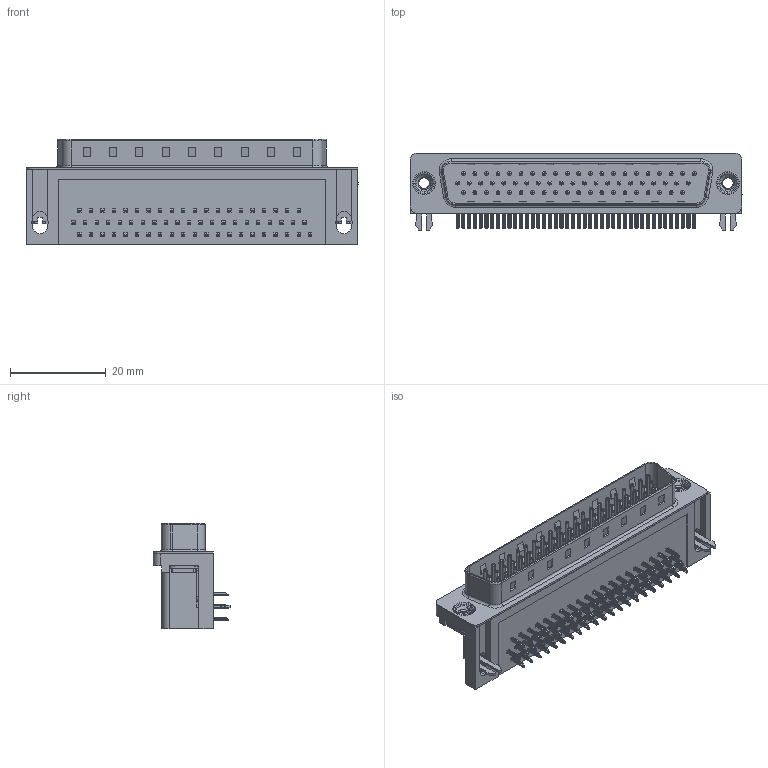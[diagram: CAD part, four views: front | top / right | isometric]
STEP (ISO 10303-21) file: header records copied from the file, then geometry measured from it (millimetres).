
FILE_DESCRIPTION (( 'STEP AP203' ), '1' );
FILE_NAME ('633-062-263-032.STEP', '2018-09-07T21:38:47', ( '' ), ( '' ), 'SwSTEP 2.0', 'SolidWorks 2016', '' );
FILE_SCHEMA (( 'CONFIG_CONTROL_DESIGN' ));
Length unit declared in the file: millimetre
Products named in the file (8): 633 2 Prong Board Lock; 633 4-40 Threaded Rivet; 633-062-263-032; 633 Housing_62 Contact; 633 Shell_62 Contact; 633 Contact Bottom; 633 Contact Middle; 633 Contact Top
Assembly tree (68 placements, depth 2):
  633-062-263-032
    633 Housing_62 Contact
    633 Shell_62 Contact
    633 Contact Bottom  x20
    633 Contact Middle  x21
    633 Contact Top  x21
    633 2 Prong Board Lock  x2
    633 4-40 Threaded Rivet  x2
Bounding box: 69.4 x 16.25 x 22.1 mm (x, y, z)
Volume: 11055 mm3; surface area: 13409.9 mm2
Topology: 68 solids, 68 shells, 5116 faces, 12606 edges, 7757 vertices
Faces by surface type: plane 3245, cylinder 1450, torus 403, cone 12, bspline 6
Entity records: 35933 total; most frequent: CARTESIAN_POINT 7291, DIRECTION 5524, ORIENTED_EDGE 5258, EDGE_CURVE 2629, LINE 1920, VECTOR 1920, AXIS2_PLACEMENT_3D 1802, VERTEX_POINT 1699
